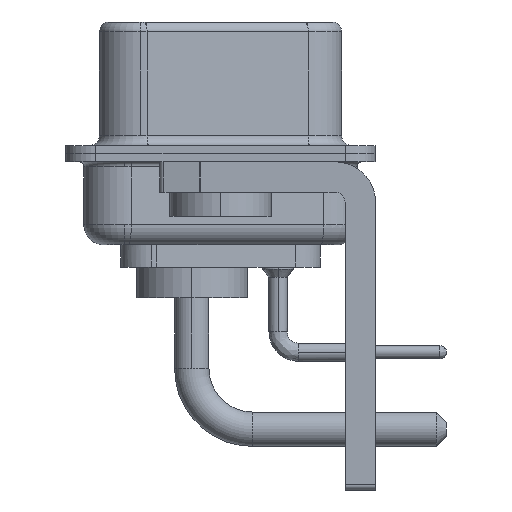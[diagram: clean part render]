
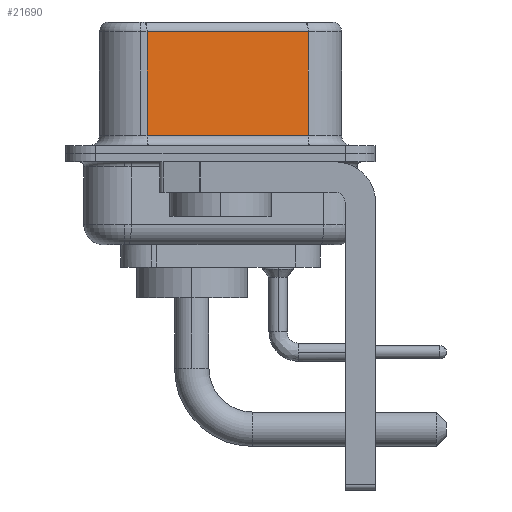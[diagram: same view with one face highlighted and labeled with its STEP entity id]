
A CAD part, left-side view. The second image highlights one B-rep face of the part: STEP entity #21690.
In plain terms, the highlighted planar face has unit normal (-0.985, -0.174, 0).
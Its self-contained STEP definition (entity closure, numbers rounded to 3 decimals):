
#456 = CARTESIAN_POINT ( 'NONE',  ( 5.132, -4.322, 0.9 ) ) ;
#726 = DIRECTION ( 'NONE',  ( -0.174, 0.985, 0. ) ) ;
#785 = EDGE_CURVE ( 'NONE', #17311, #8572, #7099, .T. ) ;
#832 = VERTEX_POINT ( 'NONE', #22899 ) ;
#1026 = AXIS2_PLACEMENT_3D ( 'NONE', #19034, #24462, #24829 ) ;
#1354 = ORIENTED_EDGE ( 'NONE', *, *, #3748, .T. ) ;
#3748 = EDGE_CURVE ( 'NONE', #22132, #832, #4159, .T. ) ;
#4159 = LINE ( 'NONE', #15344, #15669 ) ;
#4552 = CARTESIAN_POINT ( 'NONE',  ( 5.132, -4.322, 0.9 ) ) ;
#5085 = CARTESIAN_POINT ( 'NONE',  ( 5.132, -4.322, 6.52 ) ) ;
#5483 = FACE_OUTER_BOUND ( 'NONE', #20196, .T. ) ;
#5516 = VECTOR ( 'NONE', #726, 1000. ) ;
#5755 = VECTOR ( 'NONE', #20121, 1000. ) ;
#6237 = ORIENTED_EDGE ( 'NONE', *, *, #19717, .T. ) ;
#6506 = VECTOR ( 'NONE', #21917, 1000. ) ;
#7099 = LINE ( 'NONE', #5085, #6506 ) ;
#8257 = CARTESIAN_POINT ( 'NONE',  ( 5.132, -4.322, 6.02 ) ) ;
#8572 = VERTEX_POINT ( 'NONE', #456 ) ;
#9972 = EDGE_CURVE ( 'NONE', #17311, #22132, #17781, .T. ) ;
#13353 = ORIENTED_EDGE ( 'NONE', *, *, #785, .F. ) ;
#15344 = CARTESIAN_POINT ( 'NONE',  ( 3.73, 3.628, 6.52 ) ) ;
#15669 = VECTOR ( 'NONE', #22888, 1000. ) ;
#15865 = LINE ( 'NONE', #4552, #5755 ) ;
#16569 = ORIENTED_EDGE ( 'NONE', *, *, #9972, .T. ) ;
#17311 = VERTEX_POINT ( 'NONE', #24486 ) ;
#17781 = LINE ( 'NONE', #8257, #5516 ) ;
#18807 = PLANE ( 'NONE',  #1026 ) ;
#19034 = CARTESIAN_POINT ( 'NONE',  ( 5.132, -4.322, 6.52 ) ) ;
#19717 = EDGE_CURVE ( 'NONE', #832, #8572, #15865, .T. ) ;
#20121 = DIRECTION ( 'NONE',  ( 0.174, -0.985, 0. ) ) ;
#20196 = EDGE_LOOP ( 'NONE', ( #13353, #16569, #1354, #6237 ) ) ;
#21690 = ADVANCED_FACE ( 'NONE', ( #5483 ), #18807, .F. ) ;
#21917 = DIRECTION ( 'NONE',  ( 0., 0., -1. ) ) ;
#22132 = VERTEX_POINT ( 'NONE', #22293 ) ;
#22293 = CARTESIAN_POINT ( 'NONE',  ( 3.73, 3.628, 6.02 ) ) ;
#22888 = DIRECTION ( 'NONE',  ( 0., 0., -1. ) ) ;
#22899 = CARTESIAN_POINT ( 'NONE',  ( 3.73, 3.628, 0.9 ) ) ;
#24462 = DIRECTION ( 'NONE',  ( 0.985, 0.174, 0. ) ) ;
#24486 = CARTESIAN_POINT ( 'NONE',  ( 5.132, -4.322, 6.02 ) ) ;
#24829 = DIRECTION ( 'NONE',  ( -0.174, 0.985, 0. ) ) ;
